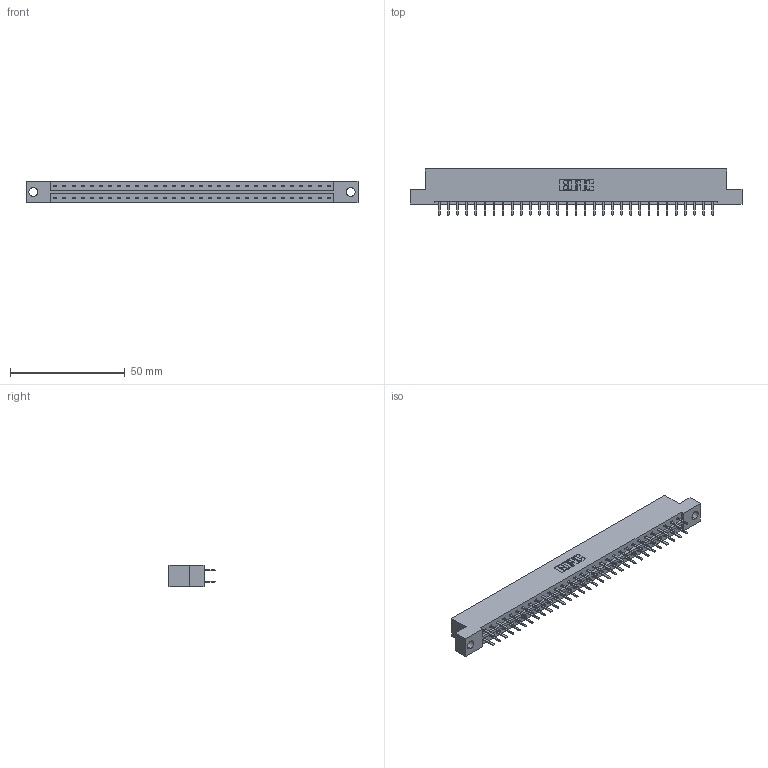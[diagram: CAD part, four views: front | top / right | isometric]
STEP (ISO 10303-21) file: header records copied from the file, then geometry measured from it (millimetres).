
FILE_DESCRIPTION (( 'STEP AP203' ), '1' );
FILE_NAME ('333-062-520-204.STEP', '2018-08-04T08:05:20', ( '' ), ( '' ), 'SwSTEP 2.0', 'SolidWorks 2016', '' );
FILE_SCHEMA (( 'CONFIG_CONTROL_DESIGN' ));
Length unit declared in the file: inch
Products named in the file (3): 333 Part_Flush - .156 Dia - TH; 345-292-001_345-293-120; 333-062-520-204
Assembly tree (63 placements, depth 2):
  333-062-520-204
    333 Part_Flush - .156 Dia - TH
    345-292-001_345-293-120  x62
Bounding box: 144.37 x 20.02 x 9.4 mm (x, y, z)
Volume: 14521.7 mm3; surface area: 16777.3 mm2
Topology: 63 solids, 63 shells, 3586 faces, 10417 edges, 6778 vertices
Faces by surface type: plane 2426, cylinder 1160
Entity records: 21483 total; most frequent: CARTESIAN_POINT 3586, ORIENTED_EDGE 3510, DIRECTION 3071, EDGE_CURVE 1755, LINE 1623, VECTOR 1623, VERTEX_POINT 1166, AXIS2_PLACEMENT_3D 724
